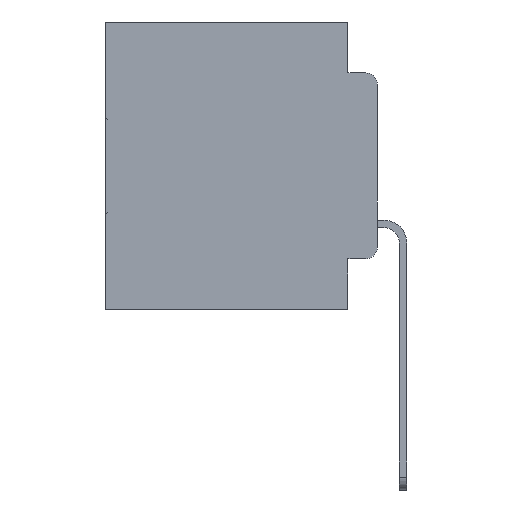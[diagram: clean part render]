
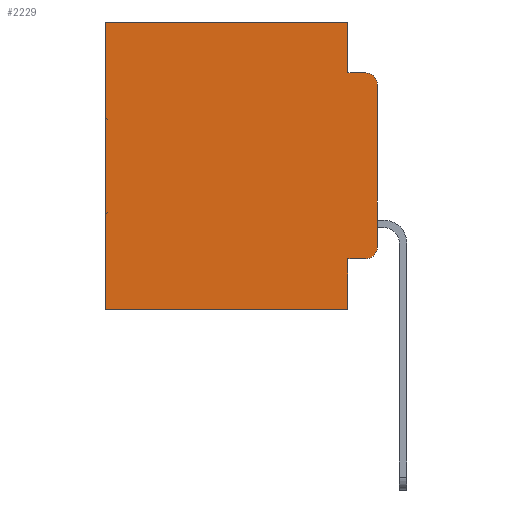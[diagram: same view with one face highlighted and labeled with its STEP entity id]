
A CAD part, left-side view. The second image highlights one B-rep face of the part: STEP entity #2229.
In plain terms, the highlighted planar face has unit normal (-1, 0, 0).
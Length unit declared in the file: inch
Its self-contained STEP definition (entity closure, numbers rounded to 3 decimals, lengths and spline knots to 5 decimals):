
#333 = ORIENTED_EDGE ( 'NONE', *, *, #5077, .F. ) ;
#495 = CIRCLE ( 'NONE', #12348, 0.02 ) ;
#1275 = ORIENTED_EDGE ( 'NONE', *, *, #15766, .T. ) ;
#2112 = DIRECTION ( 'NONE',  ( 0., 0., -1. ) ) ;
#2229 = ADVANCED_FACE ( 'NONE', ( #8937 ), #27896, .F. ) ;
#2326 = CARTESIAN_POINT ( 'NONE',  ( 0.298, 0.02, -0.1085 ) ) ;
#2750 = EDGE_CURVE ( 'NONE', #27362, #8420, #4544, .T. ) ;
#3539 = EDGE_CURVE ( 'NONE', #8420, #9588, #14686, .T. ) ;
#3718 = AXIS2_PLACEMENT_3D ( 'NONE', #32894, #17719, #2112 ) ;
#4544 = LINE ( 'NONE', #17575, #11544 ) ;
#4939 = DIRECTION ( 'NONE',  ( 0., 0., -1. ) ) ;
#5077 = EDGE_CURVE ( 'NONE', #9386, #9588, #21018, .T. ) ;
#5679 = CARTESIAN_POINT ( 'NONE',  ( 0.298, 0.02, -0.0885 ) ) ;
#5895 = VERTEX_POINT ( 'NONE', #6612 ) ;
#5951 = VECTOR ( 'NONE', #26132, 39.37008 ) ;
#6343 = DIRECTION ( 'NONE',  ( -1., 0., 0. ) ) ;
#6438 = CARTESIAN_POINT ( 'NONE',  ( 0.298, 0.051, 0. ) ) ;
#6543 = VERTEX_POINT ( 'NONE', #12421 ) ;
#6612 = CARTESIAN_POINT ( 'NONE',  ( 0.298, 0., -0.3915 ) ) ;
#7043 = EDGE_CURVE ( 'NONE', #27362, #7729, #10460, .T. ) ;
#7640 = CARTESIAN_POINT ( 'NONE',  ( 0.298, 0.473, 0. ) ) ;
#7729 = VERTEX_POINT ( 'NONE', #8140 ) ;
#7954 = CARTESIAN_POINT ( 'NONE',  ( 0.298, 0.02, -0.4115 ) ) ;
#8063 = DIRECTION ( 'NONE',  ( 0., 0., -1. ) ) ;
#8140 = CARTESIAN_POINT ( 'NONE',  ( 0.298, 0.051, -0.0885 ) ) ;
#8420 = VERTEX_POINT ( 'NONE', #16168 ) ;
#8601 = VECTOR ( 'NONE', #28275, 39.37008 ) ;
#8804 = ORIENTED_EDGE ( 'NONE', *, *, #12313, .F. ) ;
#8937 = FACE_OUTER_BOUND ( 'NONE', #23353, .T. ) ;
#9386 = VERTEX_POINT ( 'NONE', #32566 ) ;
#9588 = VERTEX_POINT ( 'NONE', #33402 ) ;
#10460 = LINE ( 'NONE', #26116, #18132 ) ;
#10692 = ORIENTED_EDGE ( 'NONE', *, *, #30100, .F. ) ;
#10990 = ORIENTED_EDGE ( 'NONE', *, *, #24355, .F. ) ;
#11169 = CARTESIAN_POINT ( 'NONE',  ( 0.298, 0., -0.5 ) ) ;
#11544 = VECTOR ( 'NONE', #22612, 39.37008 ) ;
#11584 = CARTESIAN_POINT ( 'NONE',  ( 0.298, 0., -0.1085 ) ) ;
#12007 = DIRECTION ( 'NONE',  ( 0., -1., 0. ) ) ;
#12313 = EDGE_CURVE ( 'NONE', #7729, #29384, #19700, .T. ) ;
#12348 = AXIS2_PLACEMENT_3D ( 'NONE', #2326, #20506, #4939 ) ;
#12421 = CARTESIAN_POINT ( 'NONE',  ( 0.298, 0.051, -0.4115 ) ) ;
#12617 = VERTEX_POINT ( 'NONE', #7954 ) ;
#12827 = VECTOR ( 'NONE', #12007, 39.37008 ) ;
#12899 = LINE ( 'NONE', #20981, #5951 ) ;
#13600 = VECTOR ( 'NONE', #30482, 39.37008 ) ;
#14182 = VECTOR ( 'NONE', #31306, 39.37008 ) ;
#14183 = VECTOR ( 'NONE', #16340, 39.37008 ) ;
#14386 = LINE ( 'NONE', #22936, #13600 ) ;
#14686 = LINE ( 'NONE', #7640, #8601 ) ;
#15766 = EDGE_CURVE ( 'NONE', #17613, #29384, #495, .T. ) ;
#16168 = CARTESIAN_POINT ( 'NONE',  ( 0.298, 0.473, 0. ) ) ;
#16340 = DIRECTION ( 'NONE',  ( 0., 1., 0. ) ) ;
#17170 = ORIENTED_EDGE ( 'NONE', *, *, #24992, .T. ) ;
#17575 = CARTESIAN_POINT ( 'NONE',  ( 0.298, 0., 0. ) ) ;
#17613 = VERTEX_POINT ( 'NONE', #11584 ) ;
#17719 = DIRECTION ( 'NONE',  ( 1., 0., 0. ) ) ;
#18132 = VECTOR ( 'NONE', #8063, 39.37008 ) ;
#19700 = LINE ( 'NONE', #22228, #12827 ) ;
#20136 = ORIENTED_EDGE ( 'NONE', *, *, #2750, .T. ) ;
#20506 = DIRECTION ( 'NONE',  ( -1., 0., 0. ) ) ;
#20981 = CARTESIAN_POINT ( 'NONE',  ( 0.298, 0.051, -0.4115 ) ) ;
#21018 = LINE ( 'NONE', #11169, #14183 ) ;
#21225 = CARTESIAN_POINT ( 'NONE',  ( 0.298, 0., 0. ) ) ;
#21874 = CARTESIAN_POINT ( 'NONE',  ( 0.298, 0.02, -0.3915 ) ) ;
#22228 = CARTESIAN_POINT ( 'NONE',  ( 0.298, 0.051, -0.0885 ) ) ;
#22612 = DIRECTION ( 'NONE',  ( 0., 1., 0. ) ) ;
#22936 = CARTESIAN_POINT ( 'NONE',  ( 0.298, 0.051, 0. ) ) ;
#23353 = EDGE_LOOP ( 'NONE', ( #10990, #1275, #8804, #31559, #20136, #24834, #333, #10692, #29442, #17170 ) ) ;
#24355 = EDGE_CURVE ( 'NONE', #17613, #5895, #28632, .T. ) ;
#24422 = DIRECTION ( 'NONE',  ( 0., 0., -1. ) ) ;
#24834 = ORIENTED_EDGE ( 'NONE', *, *, #3539, .T. ) ;
#24992 = EDGE_CURVE ( 'NONE', #12617, #5895, #26465, .T. ) ;
#25598 = AXIS2_PLACEMENT_3D ( 'NONE', #21874, #6343, #24422 ) ;
#26116 = CARTESIAN_POINT ( 'NONE',  ( 0.298, 0.051, 0. ) ) ;
#26132 = DIRECTION ( 'NONE',  ( 0., -1., 0. ) ) ;
#26465 = CIRCLE ( 'NONE', #25598, 0.02 ) ;
#27362 = VERTEX_POINT ( 'NONE', #6438 ) ;
#27896 = PLANE ( 'NONE',  #3718 ) ;
#28275 = DIRECTION ( 'NONE',  ( 0., 0., -1. ) ) ;
#28446 = EDGE_CURVE ( 'NONE', #6543, #12617, #12899, .T. ) ;
#28632 = LINE ( 'NONE', #21225, #14182 ) ;
#29384 = VERTEX_POINT ( 'NONE', #5679 ) ;
#29442 = ORIENTED_EDGE ( 'NONE', *, *, #28446, .T. ) ;
#30100 = EDGE_CURVE ( 'NONE', #6543, #9386, #14386, .T. ) ;
#30482 = DIRECTION ( 'NONE',  ( 0., 0., -1. ) ) ;
#31306 = DIRECTION ( 'NONE',  ( 0., 0., -1. ) ) ;
#31559 = ORIENTED_EDGE ( 'NONE', *, *, #7043, .F. ) ;
#32566 = CARTESIAN_POINT ( 'NONE',  ( 0.298, 0.051, -0.5 ) ) ;
#32894 = CARTESIAN_POINT ( 'NONE',  ( 0.298, 0., 0. ) ) ;
#33402 = CARTESIAN_POINT ( 'NONE',  ( 0.298, 0.473, -0.5 ) ) ;
